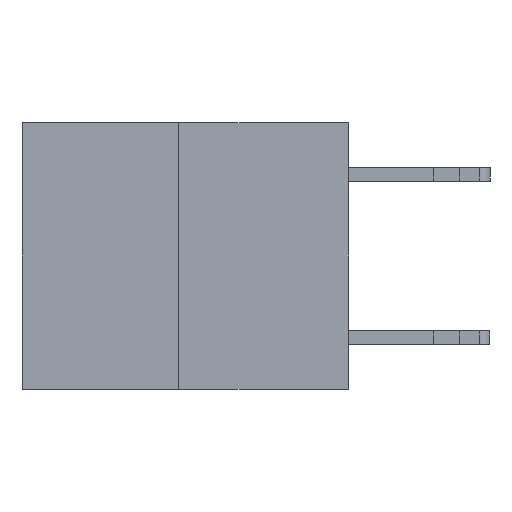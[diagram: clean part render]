
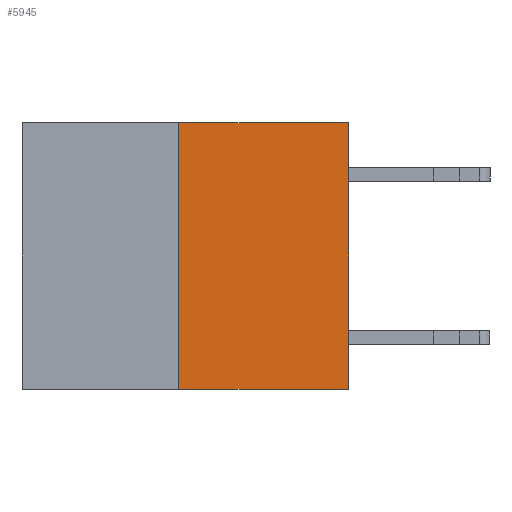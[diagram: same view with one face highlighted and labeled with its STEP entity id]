
A CAD part, left-side view. The second image highlights one B-rep face of the part: STEP entity #5945.
In plain terms, the highlighted planar face has unit normal (-1, 0, 0).
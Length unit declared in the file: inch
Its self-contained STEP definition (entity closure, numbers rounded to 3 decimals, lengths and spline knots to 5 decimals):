
#214 = AXIS2_PLACEMENT_3D ( 'NONE', #3162, #14615, #12375 ) ;
#466 = CARTESIAN_POINT ( 'NONE',  ( 0., 0., -0.49 ) ) ;
#911 = PLANE ( 'NONE',  #214 ) ;
#1268 = CARTESIAN_POINT ( 'NONE',  ( 0., 0., 0. ) ) ;
#2075 = ORIENTED_EDGE ( 'NONE', *, *, #6931, .T. ) ;
#2188 = VECTOR ( 'NONE', #9401, 39.37008 ) ;
#2633 = DIRECTION ( 'NONE',  ( 0., -1., 0. ) ) ;
#2640 = CARTESIAN_POINT ( 'NONE',  ( 0., 0.312, -0.49 ) ) ;
#2841 = EDGE_LOOP ( 'NONE', ( #12480, #9259, #2075, #8662 ) ) ;
#3162 = CARTESIAN_POINT ( 'NONE',  ( 0., 0.6, 0. ) ) ;
#3614 = EDGE_CURVE ( 'NONE', #5982, #11004, #10657, .T. ) ;
#3767 = LINE ( 'NONE', #4656, #12547 ) ;
#4039 = CARTESIAN_POINT ( 'NONE',  ( 0., 0., 0. ) ) ;
#4153 = CARTESIAN_POINT ( 'NONE',  ( 0., 0.312, -0.49 ) ) ;
#4656 = CARTESIAN_POINT ( 'NONE',  ( 0., 0.6, 0. ) ) ;
#5945 = ADVANCED_FACE ( 'NONE', ( #8669 ), #911, .F. ) ;
#5982 = VERTEX_POINT ( 'NONE', #4153 ) ;
#6931 = EDGE_CURVE ( 'NONE', #9205, #14775, #10617, .T. ) ;
#7121 = DIRECTION ( 'NONE',  ( 0., 0., 1. ) ) ;
#7673 = CARTESIAN_POINT ( 'NONE',  ( 0., 0.312, 0. ) ) ;
#8662 = ORIENTED_EDGE ( 'NONE', *, *, #13559, .F. ) ;
#8669 = FACE_OUTER_BOUND ( 'NONE', #2841, .T. ) ;
#9205 = VERTEX_POINT ( 'NONE', #466 ) ;
#9259 = ORIENTED_EDGE ( 'NONE', *, *, #13694, .T. ) ;
#9401 = DIRECTION ( 'NONE',  ( 0., 0., 1. ) ) ;
#10120 = VECTOR ( 'NONE', #7121, 39.37008 ) ;
#10617 = LINE ( 'NONE', #1268, #2188 ) ;
#10657 = LINE ( 'NONE', #2640, #10120 ) ;
#10930 = LINE ( 'NONE', #11687, #13771 ) ;
#11004 = VERTEX_POINT ( 'NONE', #7673 ) ;
#11687 = CARTESIAN_POINT ( 'NONE',  ( 0., 0.6, -0.49 ) ) ;
#12375 = DIRECTION ( 'NONE',  ( 0., 0., -1. ) ) ;
#12480 = ORIENTED_EDGE ( 'NONE', *, *, #3614, .F. ) ;
#12547 = VECTOR ( 'NONE', #13739, 39.37008 ) ;
#13559 = EDGE_CURVE ( 'NONE', #11004, #14775, #3767, .T. ) ;
#13694 = EDGE_CURVE ( 'NONE', #5982, #9205, #10930, .T. ) ;
#13739 = DIRECTION ( 'NONE',  ( 0., -1., 0. ) ) ;
#13771 = VECTOR ( 'NONE', #2633, 39.37008 ) ;
#14615 = DIRECTION ( 'NONE',  ( 1., 0., 0. ) ) ;
#14775 = VERTEX_POINT ( 'NONE', #4039 ) ;
